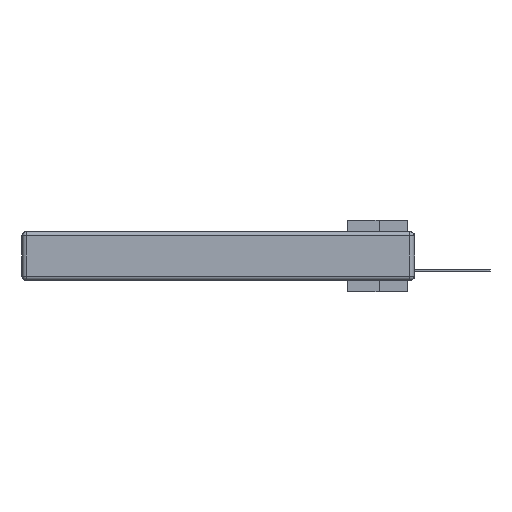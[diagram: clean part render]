
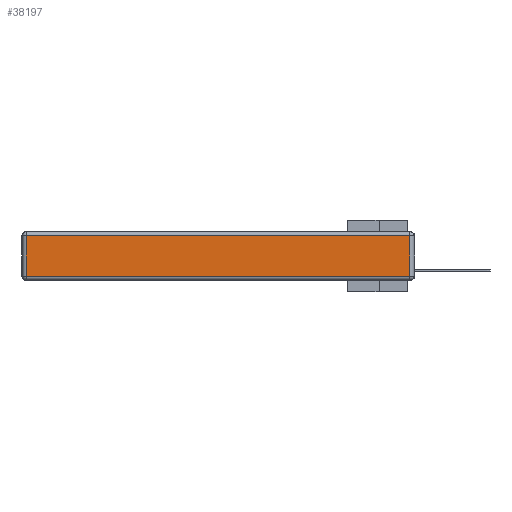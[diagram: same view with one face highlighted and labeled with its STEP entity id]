
A CAD part, left-side view. The second image highlights one B-rep face of the part: STEP entity #38197.
In plain terms, the highlighted planar face has unit normal (-1, 0, 0).
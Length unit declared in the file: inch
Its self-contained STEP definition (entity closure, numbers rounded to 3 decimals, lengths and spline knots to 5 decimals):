
#1851 = VERTEX_POINT ( 'NONE', #26635 ) ;
#1942 = ORIENTED_EDGE ( 'NONE', *, *, #21184, .T. ) ;
#2610 = AXIS2_PLACEMENT_3D ( 'NONE', #19725, #15939, #16138 ) ;
#4314 = CARTESIAN_POINT ( 'NONE',  ( 0., 0., -0.313 ) ) ;
#4416 = ORIENTED_EDGE ( 'NONE', *, *, #21660, .T. ) ;
#7377 = FACE_OUTER_BOUND ( 'NONE', #15455, .T. ) ;
#10569 = DIRECTION ( 'NONE',  ( 0., 1., 0. ) ) ;
#12918 = LINE ( 'NONE', #16283, #30522 ) ;
#13892 = VECTOR ( 'NONE', #10569, 39.37008 ) ;
#14150 = VERTEX_POINT ( 'NONE', #21922 ) ;
#15455 = EDGE_LOOP ( 'NONE', ( #30381, #4416, #1942, #26871 ) ) ;
#15731 = DIRECTION ( 'NONE',  ( 0., 0., -1. ) ) ;
#15939 = DIRECTION ( 'NONE',  ( -1., 0., 0. ) ) ;
#16138 = DIRECTION ( 'NONE',  ( 0., 0., 1. ) ) ;
#16283 = CARTESIAN_POINT ( 'NONE',  ( 0., 0.03, -0.343 ) ) ;
#16321 = LINE ( 'NONE', #19128, #13892 ) ;
#19128 = CARTESIAN_POINT ( 'NONE',  ( 0., 2.75, -0.03 ) ) ;
#19725 = CARTESIAN_POINT ( 'NONE',  ( 0., 0., -0.343 ) ) ;
#20215 = CARTESIAN_POINT ( 'NONE',  ( 0., 2.72, -0.313 ) ) ;
#21184 = EDGE_CURVE ( 'NONE', #14150, #26719, #16321, .T. ) ;
#21660 = EDGE_CURVE ( 'NONE', #1851, #14150, #12918, .T. ) ;
#21922 = CARTESIAN_POINT ( 'NONE',  ( 0., 0.03, -0.03 ) ) ;
#24951 = CARTESIAN_POINT ( 'NONE',  ( 0., 2.72, -0.343 ) ) ;
#25548 = PLANE ( 'NONE',  #2610 ) ;
#26635 = CARTESIAN_POINT ( 'NONE',  ( 0., 0.03, -0.313 ) ) ;
#26719 = VERTEX_POINT ( 'NONE', #34931 ) ;
#26871 = ORIENTED_EDGE ( 'NONE', *, *, #36951, .T. ) ;
#28508 = DIRECTION ( 'NONE',  ( 0., 0., 1. ) ) ;
#28554 = VERTEX_POINT ( 'NONE', #20215 ) ;
#28745 = LINE ( 'NONE', #24951, #31880 ) ;
#30381 = ORIENTED_EDGE ( 'NONE', *, *, #33539, .T. ) ;
#30393 = VECTOR ( 'NONE', #37851, 39.37008 ) ;
#30522 = VECTOR ( 'NONE', #28508, 39.37008 ) ;
#31880 = VECTOR ( 'NONE', #15731, 39.37008 ) ;
#33539 = EDGE_CURVE ( 'NONE', #28554, #1851, #38036, .T. ) ;
#34931 = CARTESIAN_POINT ( 'NONE',  ( 0., 2.72, -0.03 ) ) ;
#36951 = EDGE_CURVE ( 'NONE', #26719, #28554, #28745, .T. ) ;
#37851 = DIRECTION ( 'NONE',  ( 0., -1., 0. ) ) ;
#38036 = LINE ( 'NONE', #4314, #30393 ) ;
#38197 = ADVANCED_FACE ( 'NONE', ( #7377 ), #25548, .T. ) ;
